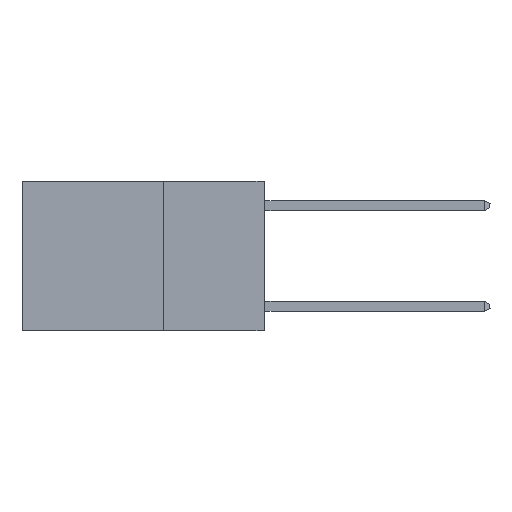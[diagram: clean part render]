
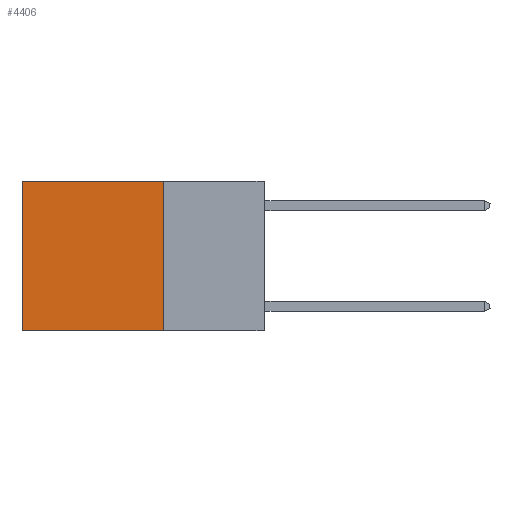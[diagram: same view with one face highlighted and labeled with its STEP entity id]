
A CAD part, left-side view. The second image highlights one B-rep face of the part: STEP entity #4406.
In plain terms, the highlighted planar face has unit normal (-1, 0, 0).
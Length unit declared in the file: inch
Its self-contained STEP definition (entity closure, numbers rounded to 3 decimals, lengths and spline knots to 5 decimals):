
#1178 = DIRECTION ( 'NONE',  ( 0., 0., -1. ) ) ;
#1297 = CARTESIAN_POINT ( 'NONE',  ( 0.2625, 0.25, -0.37 ) ) ;
#1301 = LINE ( 'NONE', #13316, #12314 ) ;
#1859 = FACE_OUTER_BOUND ( 'NONE', #13169, .T. ) ;
#2627 = CARTESIAN_POINT ( 'NONE',  ( 0.2625, 0.25, 0. ) ) ;
#4406 = ADVANCED_FACE ( 'NONE', ( #1859 ), #13869, .F. ) ;
#4974 = CARTESIAN_POINT ( 'NONE',  ( 0.2625, 0.25, 0. ) ) ;
#5347 = CARTESIAN_POINT ( 'NONE',  ( 0.2625, 0.25, 0. ) ) ;
#5992 = VECTOR ( 'NONE', #8229, 39.37008 ) ;
#6385 = VERTEX_POINT ( 'NONE', #2627 ) ;
#6504 = EDGE_CURVE ( 'NONE', #6385, #15094, #15182, .T. ) ;
#8208 = EDGE_CURVE ( 'NONE', #6385, #17039, #14975, .T. ) ;
#8229 = DIRECTION ( 'NONE',  ( 0., 1., 0. ) ) ;
#9729 = AXIS2_PLACEMENT_3D ( 'NONE', #5347, #10052, #18701 ) ;
#10052 = DIRECTION ( 'NONE',  ( 1., 0., 0. ) ) ;
#10102 = VERTEX_POINT ( 'NONE', #20372 ) ;
#11161 = CARTESIAN_POINT ( 'NONE',  ( 0.2625, 0.6, 0. ) ) ;
#11210 = DIRECTION ( 'NONE',  ( 0., 1., 0. ) ) ;
#11883 = ORIENTED_EDGE ( 'NONE', *, *, #12632, .T. ) ;
#12314 = VECTOR ( 'NONE', #11210, 39.37008 ) ;
#12632 = EDGE_CURVE ( 'NONE', #15094, #10102, #19591, .T. ) ;
#12638 = CARTESIAN_POINT ( 'NONE',  ( 0.2625, 0.6, 0. ) ) ;
#12814 = VECTOR ( 'NONE', #1178, 39.37008 ) ;
#13169 = EDGE_LOOP ( 'NONE', ( #11883, #16963, #18817, #15762 ) ) ;
#13316 = CARTESIAN_POINT ( 'NONE',  ( 0.2625, 0.25, -0.37 ) ) ;
#13411 = DIRECTION ( 'NONE',  ( 0., 0., -1. ) ) ;
#13869 = PLANE ( 'NONE',  #9729 ) ;
#14975 = LINE ( 'NONE', #16896, #16068 ) ;
#15094 = VERTEX_POINT ( 'NONE', #12638 ) ;
#15182 = LINE ( 'NONE', #4974, #5992 ) ;
#15762 = ORIENTED_EDGE ( 'NONE', *, *, #6504, .T. ) ;
#16068 = VECTOR ( 'NONE', #13411, 39.37008 ) ;
#16896 = CARTESIAN_POINT ( 'NONE',  ( 0.2625, 0.25, 0. ) ) ;
#16963 = ORIENTED_EDGE ( 'NONE', *, *, #18436, .F. ) ;
#17039 = VERTEX_POINT ( 'NONE', #1297 ) ;
#18436 = EDGE_CURVE ( 'NONE', #17039, #10102, #1301, .T. ) ;
#18701 = DIRECTION ( 'NONE',  ( 0., 0., -1. ) ) ;
#18817 = ORIENTED_EDGE ( 'NONE', *, *, #8208, .F. ) ;
#19591 = LINE ( 'NONE', #11161, #12814 ) ;
#20372 = CARTESIAN_POINT ( 'NONE',  ( 0.2625, 0.6, -0.37 ) ) ;
